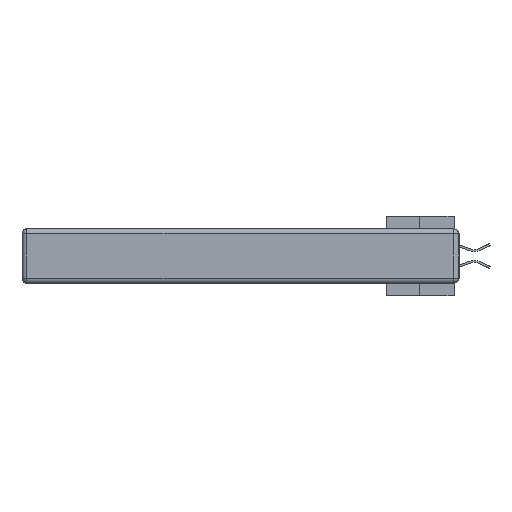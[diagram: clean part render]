
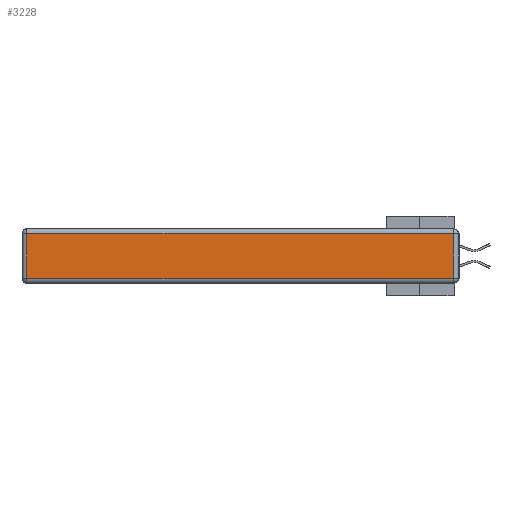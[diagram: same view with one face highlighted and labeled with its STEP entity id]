
A CAD part, left-side view. The second image highlights one B-rep face of the part: STEP entity #3228.
In plain terms, the highlighted planar face has unit normal (-1, 0, 0).
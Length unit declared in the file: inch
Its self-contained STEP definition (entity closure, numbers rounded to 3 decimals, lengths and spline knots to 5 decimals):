
#303 = CARTESIAN_POINT ( 'NONE',  ( 0., 0.03, -0.343 ) ) ;
#3228 = ADVANCED_FACE ( 'NONE', ( #11388 ), #15809, .T. ) ;
#5319 = CARTESIAN_POINT ( 'NONE',  ( 0., 0.03, -0.313 ) ) ;
#5520 = CARTESIAN_POINT ( 'NONE',  ( 0., 0.03, -0.03 ) ) ;
#5767 = ORIENTED_EDGE ( 'NONE', *, *, #40295, .T. ) ;
#6418 = VECTOR ( 'NONE', #10007, 39.37008 ) ;
#8081 = ORIENTED_EDGE ( 'NONE', *, *, #41026, .T. ) ;
#10007 = DIRECTION ( 'NONE',  ( 0., 0., 1. ) ) ;
#10917 = VECTOR ( 'NONE', #19084, 39.37008 ) ;
#11181 = CARTESIAN_POINT ( 'NONE',  ( 0., 2.75, -0.03 ) ) ;
#11388 = FACE_OUTER_BOUND ( 'NONE', #30397, .T. ) ;
#11433 = LINE ( 'NONE', #11181, #10917 ) ;
#12969 = VERTEX_POINT ( 'NONE', #5319 ) ;
#14698 = CARTESIAN_POINT ( 'NONE',  ( 0., 2.72, -0.03 ) ) ;
#14795 = VERTEX_POINT ( 'NONE', #37670 ) ;
#15809 = PLANE ( 'NONE',  #32406 ) ;
#15956 = CARTESIAN_POINT ( 'NONE',  ( 0., 0., -0.343 ) ) ;
#17520 = VECTOR ( 'NONE', #28736, 39.37008 ) ;
#19084 = DIRECTION ( 'NONE',  ( 0., 1., 0. ) ) ;
#19192 = DIRECTION ( 'NONE',  ( -1., 0., 0. ) ) ;
#21208 = VECTOR ( 'NONE', #36737, 39.37008 ) ;
#21723 = CARTESIAN_POINT ( 'NONE',  ( 0., 2.72, -0.343 ) ) ;
#23522 = CARTESIAN_POINT ( 'NONE',  ( 0., 0., -0.313 ) ) ;
#25620 = LINE ( 'NONE', #21723, #17520 ) ;
#27570 = ORIENTED_EDGE ( 'NONE', *, *, #38495, .T. ) ;
#28736 = DIRECTION ( 'NONE',  ( 0., 0., -1. ) ) ;
#30313 = VERTEX_POINT ( 'NONE', #5520 ) ;
#30397 = EDGE_LOOP ( 'NONE', ( #27570, #8081, #5767, #40192 ) ) ;
#31118 = LINE ( 'NONE', #303, #6418 ) ;
#31307 = LINE ( 'NONE', #23522, #21208 ) ;
#32406 = AXIS2_PLACEMENT_3D ( 'NONE', #15956, #19192, #41709 ) ;
#33497 = EDGE_CURVE ( 'NONE', #37382, #14795, #25620, .T. ) ;
#36737 = DIRECTION ( 'NONE',  ( 0., -1., 0. ) ) ;
#37382 = VERTEX_POINT ( 'NONE', #14698 ) ;
#37670 = CARTESIAN_POINT ( 'NONE',  ( 0., 2.72, -0.313 ) ) ;
#38495 = EDGE_CURVE ( 'NONE', #14795, #12969, #31307, .T. ) ;
#40192 = ORIENTED_EDGE ( 'NONE', *, *, #33497, .T. ) ;
#40295 = EDGE_CURVE ( 'NONE', #30313, #37382, #11433, .T. ) ;
#41026 = EDGE_CURVE ( 'NONE', #12969, #30313, #31118, .T. ) ;
#41709 = DIRECTION ( 'NONE',  ( 0., 0., 1. ) ) ;
